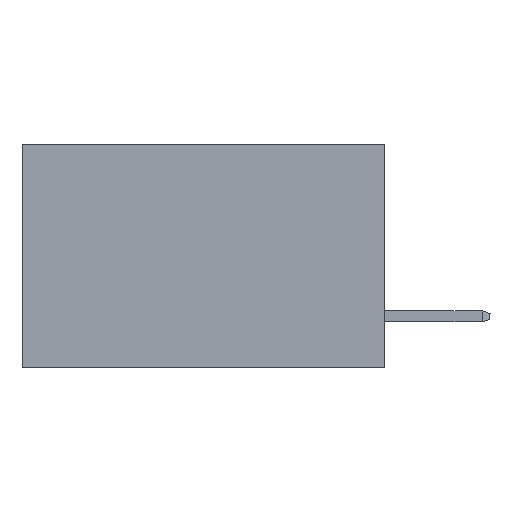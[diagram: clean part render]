
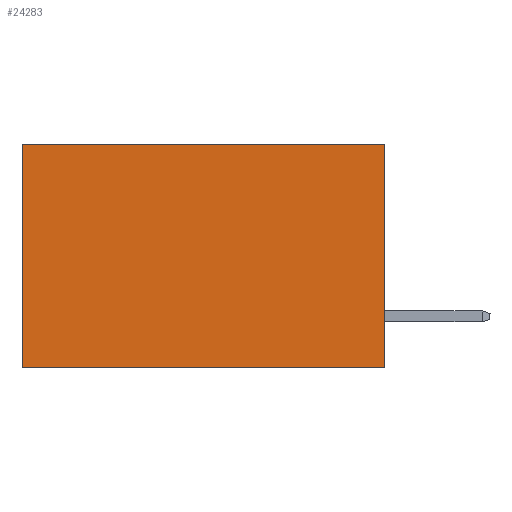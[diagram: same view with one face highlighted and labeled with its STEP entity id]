
A CAD part, left-side view. The second image highlights one B-rep face of the part: STEP entity #24283.
In plain terms, the highlighted planar face has unit normal (-1, 0, 0).
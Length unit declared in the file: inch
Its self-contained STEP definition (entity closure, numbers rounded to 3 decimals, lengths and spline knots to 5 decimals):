
#434 = EDGE_CURVE ( 'NONE', #15830, #13613, #21113, .T. ) ;
#719 = CARTESIAN_POINT ( 'NONE',  ( 0.298, 0., -0.37 ) ) ;
#1069 = AXIS2_PLACEMENT_3D ( 'NONE', #5563, #14670, #5436 ) ;
#3455 = VECTOR ( 'NONE', #3637, 39.37008 ) ;
#3637 = DIRECTION ( 'NONE',  ( 0., 0., -1. ) ) ;
#3993 = ORIENTED_EDGE ( 'NONE', *, *, #434, .F. ) ;
#4562 = DIRECTION ( 'NONE',  ( 0., 1., 0. ) ) ;
#5436 = DIRECTION ( 'NONE',  ( 0., 0., -1. ) ) ;
#5563 = CARTESIAN_POINT ( 'NONE',  ( 0.298, 0., 0. ) ) ;
#5938 = CARTESIAN_POINT ( 'NONE',  ( 0.298, 0., 0. ) ) ;
#5975 = LINE ( 'NONE', #23609, #25271 ) ;
#7460 = EDGE_LOOP ( 'NONE', ( #26655, #26459, #3993, #14460 ) ) ;
#8190 = CARTESIAN_POINT ( 'NONE',  ( 0.298, 0., 0. ) ) ;
#9114 = DIRECTION ( 'NONE',  ( 0., 1., 0. ) ) ;
#10599 = DIRECTION ( 'NONE',  ( 0., 0., -1. ) ) ;
#11052 = LINE ( 'NONE', #19866, #15755 ) ;
#12176 = VERTEX_POINT ( 'NONE', #19229 ) ;
#13539 = EDGE_CURVE ( 'NONE', #13613, #15031, #13730, .T. ) ;
#13613 = VERTEX_POINT ( 'NONE', #18353 ) ;
#13730 = LINE ( 'NONE', #719, #14613 ) ;
#14460 = ORIENTED_EDGE ( 'NONE', *, *, #21161, .T. ) ;
#14557 = EDGE_CURVE ( 'NONE', #12176, #15031, #5975, .T. ) ;
#14613 = VECTOR ( 'NONE', #9114, 39.37008 ) ;
#14670 = DIRECTION ( 'NONE',  ( 1., 0., 0. ) ) ;
#15031 = VERTEX_POINT ( 'NONE', #28205 ) ;
#15755 = VECTOR ( 'NONE', #4562, 39.37008 ) ;
#15830 = VERTEX_POINT ( 'NONE', #8190 ) ;
#16981 = PLANE ( 'NONE',  #1069 ) ;
#18353 = CARTESIAN_POINT ( 'NONE',  ( 0.298, 0., -0.37 ) ) ;
#19229 = CARTESIAN_POINT ( 'NONE',  ( 0.298, 0.6, 0. ) ) ;
#19866 = CARTESIAN_POINT ( 'NONE',  ( 0.298, 0., 0. ) ) ;
#21113 = LINE ( 'NONE', #5938, #3455 ) ;
#21161 = EDGE_CURVE ( 'NONE', #15830, #12176, #11052, .T. ) ;
#23609 = CARTESIAN_POINT ( 'NONE',  ( 0.298, 0.6, 0. ) ) ;
#24283 = ADVANCED_FACE ( 'NONE', ( #25807 ), #16981, .F. ) ;
#25271 = VECTOR ( 'NONE', #10599, 39.37008 ) ;
#25807 = FACE_OUTER_BOUND ( 'NONE', #7460, .T. ) ;
#26459 = ORIENTED_EDGE ( 'NONE', *, *, #13539, .F. ) ;
#26655 = ORIENTED_EDGE ( 'NONE', *, *, #14557, .T. ) ;
#28205 = CARTESIAN_POINT ( 'NONE',  ( 0.298, 0.6, -0.37 ) ) ;
